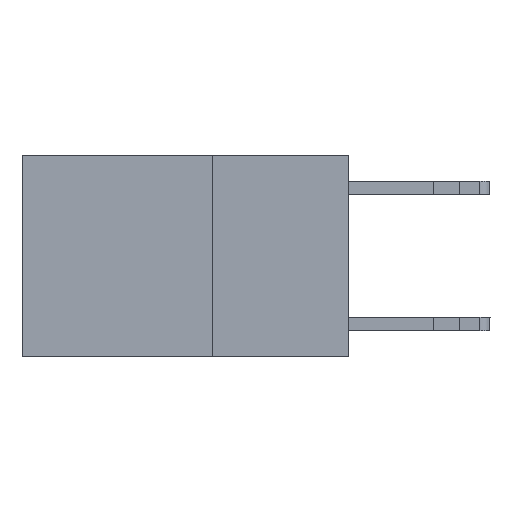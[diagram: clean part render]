
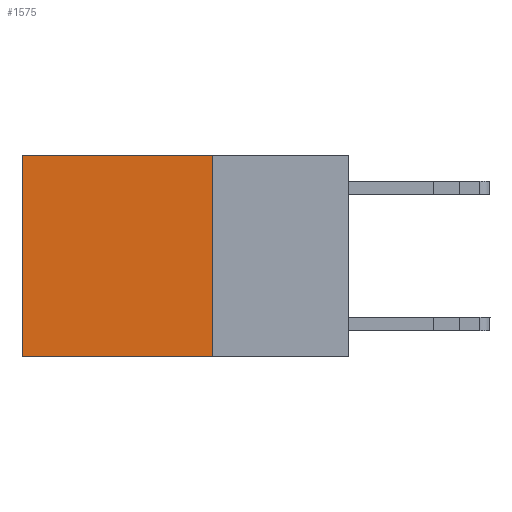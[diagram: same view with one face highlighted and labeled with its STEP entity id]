
A CAD part, left-side view. The second image highlights one B-rep face of the part: STEP entity #1575.
In plain terms, the highlighted planar face has unit normal (-1, 0, 0).
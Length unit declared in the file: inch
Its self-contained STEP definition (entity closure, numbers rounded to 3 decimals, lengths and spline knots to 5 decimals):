
#28 = DIRECTION ( 'NONE',  ( 0., 0., -1. ) ) ;
#240 = DIRECTION ( 'NONE',  ( 0., 0., -1. ) ) ;
#1275 = CARTESIAN_POINT ( 'NONE',  ( 0.2625, 0.25, 0. ) ) ;
#1575 = ADVANCED_FACE ( 'NONE', ( #8401 ), #8649, .F. ) ;
#1585 = VECTOR ( 'NONE', #18816, 39.37008 ) ;
#2337 = LINE ( 'NONE', #2820, #9211 ) ;
#2719 = VERTEX_POINT ( 'NONE', #1275 ) ;
#2820 = CARTESIAN_POINT ( 'NONE',  ( 0.2625, 0.25, 0. ) ) ;
#4529 = ORIENTED_EDGE ( 'NONE', *, *, #18692, .F. ) ;
#4702 = CARTESIAN_POINT ( 'NONE',  ( 0.2625, 0.6, 0. ) ) ;
#5299 = AXIS2_PLACEMENT_3D ( 'NONE', #9027, #10526, #240 ) ;
#6345 = EDGE_CURVE ( 'NONE', #2719, #15977, #14582, .T. ) ;
#6555 = ORIENTED_EDGE ( 'NONE', *, *, #18933, .T. ) ;
#6608 = EDGE_LOOP ( 'NONE', ( #14973, #4529, #8888, #6555 ) ) ;
#8401 = FACE_OUTER_BOUND ( 'NONE', #6608, .T. ) ;
#8601 = VERTEX_POINT ( 'NONE', #4702 ) ;
#8649 = PLANE ( 'NONE',  #5299 ) ;
#8888 = ORIENTED_EDGE ( 'NONE', *, *, #6345, .F. ) ;
#8903 = VERTEX_POINT ( 'NONE', #10109 ) ;
#9027 = CARTESIAN_POINT ( 'NONE',  ( 0.2625, 0.25, 0. ) ) ;
#9211 = VECTOR ( 'NONE', #19365, 39.37008 ) ;
#10109 = CARTESIAN_POINT ( 'NONE',  ( 0.2625, 0.6, -0.37 ) ) ;
#10413 = LINE ( 'NONE', #14457, #1585 ) ;
#10526 = DIRECTION ( 'NONE',  ( 1., 0., 0. ) ) ;
#10985 = LINE ( 'NONE', #14005, #18346 ) ;
#12929 = CARTESIAN_POINT ( 'NONE',  ( 0.2625, 0.25, -0.37 ) ) ;
#14005 = CARTESIAN_POINT ( 'NONE',  ( 0.2625, 0.6, 0. ) ) ;
#14457 = CARTESIAN_POINT ( 'NONE',  ( 0.2625, 0.25, -0.37 ) ) ;
#14582 = LINE ( 'NONE', #16416, #15735 ) ;
#14973 = ORIENTED_EDGE ( 'NONE', *, *, #18484, .T. ) ;
#15735 = VECTOR ( 'NONE', #17868, 39.37008 ) ;
#15977 = VERTEX_POINT ( 'NONE', #12929 ) ;
#16416 = CARTESIAN_POINT ( 'NONE',  ( 0.2625, 0.25, 0. ) ) ;
#17868 = DIRECTION ( 'NONE',  ( 0., 0., -1. ) ) ;
#18346 = VECTOR ( 'NONE', #28, 39.37008 ) ;
#18484 = EDGE_CURVE ( 'NONE', #8601, #8903, #10985, .T. ) ;
#18692 = EDGE_CURVE ( 'NONE', #15977, #8903, #10413, .T. ) ;
#18816 = DIRECTION ( 'NONE',  ( 0., 1., 0. ) ) ;
#18933 = EDGE_CURVE ( 'NONE', #2719, #8601, #2337, .T. ) ;
#19365 = DIRECTION ( 'NONE',  ( 0., 1., 0. ) ) ;
